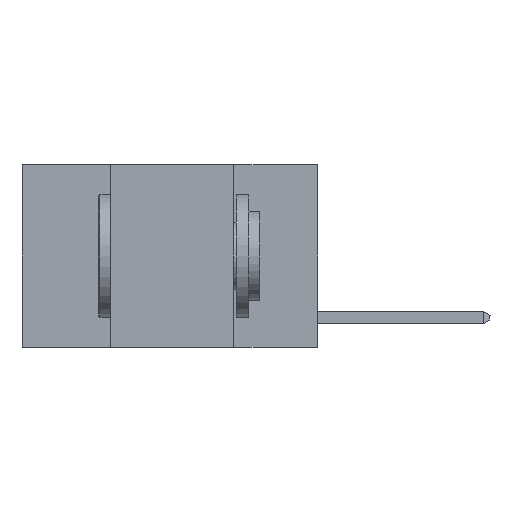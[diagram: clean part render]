
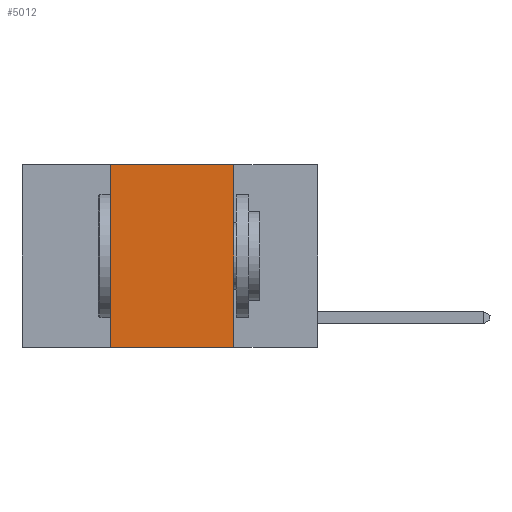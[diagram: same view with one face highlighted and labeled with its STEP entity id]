
A CAD part, left-side view. The second image highlights one B-rep face of the part: STEP entity #5012.
In plain terms, the highlighted planar face has unit normal (-1, 0, 0).
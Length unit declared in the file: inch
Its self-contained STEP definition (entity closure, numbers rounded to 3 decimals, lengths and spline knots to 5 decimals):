
#1012 = ORIENTED_EDGE ( 'NONE', *, *, #9698, .F. ) ;
#1252 = CARTESIAN_POINT ( 'NONE',  ( 0., 0.42, 0. ) ) ;
#3266 = CARTESIAN_POINT ( 'NONE',  ( 0., 0.42, 0. ) ) ;
#4234 = LINE ( 'NONE', #15622, #9761 ) ;
#4886 = ORIENTED_EDGE ( 'NONE', *, *, #14070, .T. ) ;
#5012 = ADVANCED_FACE ( 'NONE', ( #13335 ), #14365, .F. ) ;
#5466 = LINE ( 'NONE', #18341, #9802 ) ;
#5478 = VECTOR ( 'NONE', #8748, 39.37008 ) ;
#5722 = EDGE_CURVE ( 'NONE', #12091, #9177, #5466, .T. ) ;
#6357 = AXIS2_PLACEMENT_3D ( 'NONE', #13050, #7497, #7592 ) ;
#6573 = ORIENTED_EDGE ( 'NONE', *, *, #5722, .F. ) ;
#7066 = CARTESIAN_POINT ( 'NONE',  ( 0., 0.17, 0. ) ) ;
#7497 = DIRECTION ( 'NONE',  ( 1., 0., 0. ) ) ;
#7592 = DIRECTION ( 'NONE',  ( 0., 0., -1. ) ) ;
#8282 = VERTEX_POINT ( 'NONE', #13849 ) ;
#8487 = VERTEX_POINT ( 'NONE', #17114 ) ;
#8748 = DIRECTION ( 'NONE',  ( 0., 0., -1. ) ) ;
#8845 = VECTOR ( 'NONE', #18417, 39.37008 ) ;
#9177 = VERTEX_POINT ( 'NONE', #9555 ) ;
#9555 = CARTESIAN_POINT ( 'NONE',  ( 0., 0.17, 0. ) ) ;
#9698 = EDGE_CURVE ( 'NONE', #9177, #8487, #15715, .T. ) ;
#9761 = VECTOR ( 'NONE', #14108, 39.37008 ) ;
#9802 = VECTOR ( 'NONE', #11194, 39.37008 ) ;
#9816 = ORIENTED_EDGE ( 'NONE', *, *, #11505, .F. ) ;
#11194 = DIRECTION ( 'NONE',  ( 0., -1., 0. ) ) ;
#11505 = EDGE_CURVE ( 'NONE', #8282, #12091, #13067, .T. ) ;
#12091 = VERTEX_POINT ( 'NONE', #3266 ) ;
#13050 = CARTESIAN_POINT ( 'NONE',  ( 0., 0.6, 0. ) ) ;
#13067 = LINE ( 'NONE', #1252, #8845 ) ;
#13335 = FACE_OUTER_BOUND ( 'NONE', #18463, .T. ) ;
#13849 = CARTESIAN_POINT ( 'NONE',  ( 0., 0.42, -0.37 ) ) ;
#14070 = EDGE_CURVE ( 'NONE', #8282, #8487, #4234, .T. ) ;
#14108 = DIRECTION ( 'NONE',  ( 0., -1., 0. ) ) ;
#14365 = PLANE ( 'NONE',  #6357 ) ;
#15622 = CARTESIAN_POINT ( 'NONE',  ( 0., 0.6, -0.37 ) ) ;
#15715 = LINE ( 'NONE', #7066, #5478 ) ;
#17114 = CARTESIAN_POINT ( 'NONE',  ( 0., 0.17, -0.37 ) ) ;
#18341 = CARTESIAN_POINT ( 'NONE',  ( 0., 0.6, 0. ) ) ;
#18417 = DIRECTION ( 'NONE',  ( 0., 0., 1. ) ) ;
#18463 = EDGE_LOOP ( 'NONE', ( #1012, #6573, #9816, #4886 ) ) ;
